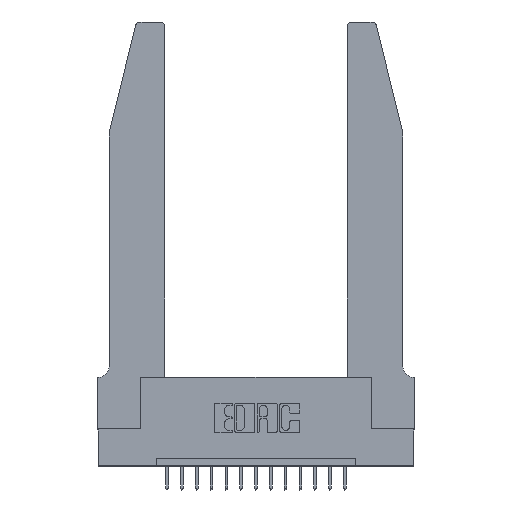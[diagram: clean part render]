
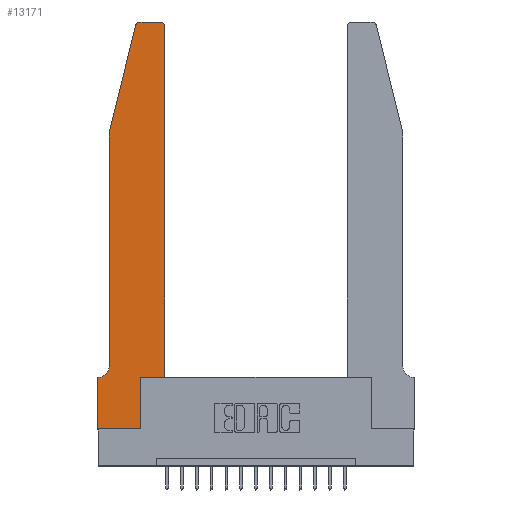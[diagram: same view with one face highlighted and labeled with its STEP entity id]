
A CAD part, top view. The second image highlights one B-rep face of the part: STEP entity #13171.
In plain terms, the highlighted planar face has unit normal (0, 0, 1).
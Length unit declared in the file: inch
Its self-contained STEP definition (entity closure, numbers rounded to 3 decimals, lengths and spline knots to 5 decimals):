
#63 = ORIENTED_EDGE ( 'NONE', *, *, #3996, .T. ) ;
#322 = FACE_OUTER_BOUND ( 'NONE', #7025, .T. ) ;
#660 = EDGE_CURVE ( 'NONE', #3453, #703, #4772, .T. ) ;
#703 = VERTEX_POINT ( 'NONE', #13868 ) ;
#1076 = VERTEX_POINT ( 'NONE', #10094 ) ;
#1338 = CARTESIAN_POINT ( 'NONE',  ( 0.0755, 2., 0.37 ) ) ;
#1634 = ORIENTED_EDGE ( 'NONE', *, *, #14730, .T. ) ;
#1838 = DIRECTION ( 'NONE',  ( 0., 1., 0. ) ) ;
#2089 = EDGE_CURVE ( 'NONE', #10853, #3168, #15451, .T. ) ;
#2152 = CARTESIAN_POINT ( 'NONE',  ( 0.4505, 0.35, 0.37 ) ) ;
#2156 = CARTESIAN_POINT ( 'NONE',  ( 0.4505, 0.35, 0.37 ) ) ;
#2313 = VECTOR ( 'NONE', #9971, 39.37008 ) ;
#2449 = DIRECTION ( 'NONE',  ( 0., 0., 1. ) ) ;
#2515 = LINE ( 'NONE', #1338, #14094 ) ;
#2856 = DIRECTION ( 'NONE',  ( 0., 0., 1. ) ) ;
#2957 = EDGE_CURVE ( 'NONE', #16217, #2970, #8934, .T. ) ;
#2970 = VERTEX_POINT ( 'NONE', #7116 ) ;
#3040 = PLANE ( 'NONE',  #16003 ) ;
#3168 = VERTEX_POINT ( 'NONE', #15044 ) ;
#3453 = VERTEX_POINT ( 'NONE', #18419 ) ;
#3845 = ORIENTED_EDGE ( 'NONE', *, *, #8795, .T. ) ;
#3909 = DIRECTION ( 'NONE',  ( 0., 0., 1. ) ) ;
#3985 = CARTESIAN_POINT ( 'NONE',  ( 0.0755, 0.35, 0.37 ) ) ;
#3996 = EDGE_CURVE ( 'NONE', #17017, #3453, #8462, .T. ) ;
#4078 = VECTOR ( 'NONE', #12708, 39.37008 ) ;
#4136 = DIRECTION ( 'NONE',  ( 0., -1., 0. ) ) ;
#4140 = LINE ( 'NONE', #13103, #18165 ) ;
#4772 = CIRCLE ( 'NONE', #15801, 0.03 ) ;
#5341 = EDGE_CURVE ( 'NONE', #1076, #16217, #13774, .T. ) ;
#5380 = CARTESIAN_POINT ( 'NONE',  ( 0.284, 2.72, 0.37 ) ) ;
#5930 = VECTOR ( 'NONE', #4136, 39.37008 ) ;
#5933 = DIRECTION ( 'NONE',  ( 1., 0., 0. ) ) ;
#6638 = DIRECTION ( 'NONE',  ( -1., 0., 0. ) ) ;
#6712 = CIRCLE ( 'NONE', #10894, 0.03 ) ;
#7025 = EDGE_LOOP ( 'NONE', ( #63, #17646, #1634, #7705, #10100, #3845, #17306, #12698, #14136, #13927, #10715, #9337 ) ) ;
#7116 = CARTESIAN_POINT ( 'NONE',  ( 0.4505, 2.72, 0.37 ) ) ;
#7169 = EDGE_CURVE ( 'NONE', #14162, #17605, #16854, .T. ) ;
#7196 = EDGE_CURVE ( 'NONE', #9338, #14162, #16417, .T. ) ;
#7284 = CARTESIAN_POINT ( 'NONE',  ( 0., 0.35, 0.37 ) ) ;
#7455 = CARTESIAN_POINT ( 'NONE',  ( 0.0755, 2., 0.37 ) ) ;
#7551 = CARTESIAN_POINT ( 'NONE',  ( 0.2605, 2.75, 0.37 ) ) ;
#7705 = ORIENTED_EDGE ( 'NONE', *, *, #7196, .T. ) ;
#8172 = DIRECTION ( 'NONE',  ( 1., 0., 0. ) ) ;
#8305 = DIRECTION ( 'NONE',  ( 1., 0., 0. ) ) ;
#8462 = LINE ( 'NONE', #7551, #4078 ) ;
#8795 = EDGE_CURVE ( 'NONE', #17605, #13874, #14074, .T. ) ;
#8934 = LINE ( 'NONE', #17096, #2313 ) ;
#9181 = VECTOR ( 'NONE', #8172, 39.37008 ) ;
#9291 = CARTESIAN_POINT ( 'NONE',  ( 0.0755, 2., 0.37 ) ) ;
#9337 = ORIENTED_EDGE ( 'NONE', *, *, #15269, .T. ) ;
#9338 = VERTEX_POINT ( 'NONE', #7455 ) ;
#9533 = CARTESIAN_POINT ( 'NONE',  ( 0.0055, 0.35, 0.37 ) ) ;
#9971 = DIRECTION ( 'NONE',  ( 0., 1., 0. ) ) ;
#10094 = CARTESIAN_POINT ( 'NONE',  ( 0.2865, 0.35, 0.37 ) ) ;
#10100 = ORIENTED_EDGE ( 'NONE', *, *, #7169, .T. ) ;
#10242 = CARTESIAN_POINT ( 'NONE',  ( 0., 0., 0.37 ) ) ;
#10715 = ORIENTED_EDGE ( 'NONE', *, *, #2957, .T. ) ;
#10853 = VERTEX_POINT ( 'NONE', #10242 ) ;
#10894 = AXIS2_PLACEMENT_3D ( 'NONE', #11143, #3909, #13817 ) ;
#11143 = CARTESIAN_POINT ( 'NONE',  ( 0.4205, 2.72, 0.37 ) ) ;
#11272 = CARTESIAN_POINT ( 'NONE',  ( 0.4205, 2.75, 0.37 ) ) ;
#11294 = DIRECTION ( 'NONE',  ( -0.239, -0.971, 0. ) ) ;
#11436 = CARTESIAN_POINT ( 'NONE',  ( 0., 0.35, 0.37 ) ) ;
#11869 = VECTOR ( 'NONE', #1838, 39.37008 ) ;
#11951 = AXIS2_PLACEMENT_3D ( 'NONE', #15025, #15149, #6638 ) ;
#12335 = LINE ( 'NONE', #14653, #11869 ) ;
#12698 = ORIENTED_EDGE ( 'NONE', *, *, #2089, .T. ) ;
#12708 = DIRECTION ( 'NONE',  ( -1., 0., 0. ) ) ;
#12768 = CARTESIAN_POINT ( 'NONE',  ( 0.0755, 0.42, 0.37 ) ) ;
#13103 = CARTESIAN_POINT ( 'NONE',  ( 0., 0., 0.37 ) ) ;
#13171 = ADVANCED_FACE ( 'NONE', ( #322 ), #3040, .T. ) ;
#13179 = VECTOR ( 'NONE', #18378, 39.37008 ) ;
#13774 = LINE ( 'NONE', #2152, #15765 ) ;
#13817 = DIRECTION ( 'NONE',  ( 1., 0., 0. ) ) ;
#13868 = CARTESIAN_POINT ( 'NONE',  ( 0.25487, 2.72718, 0.37 ) ) ;
#13874 = VERTEX_POINT ( 'NONE', #11436 ) ;
#13927 = ORIENTED_EDGE ( 'NONE', *, *, #5341, .T. ) ;
#14074 = LINE ( 'NONE', #3985, #13179 ) ;
#14094 = VECTOR ( 'NONE', #11294, 39.37008 ) ;
#14108 = CARTESIAN_POINT ( 'NONE',  ( 0., 0., 0.37 ) ) ;
#14136 = ORIENTED_EDGE ( 'NONE', *, *, #14348, .T. ) ;
#14162 = VERTEX_POINT ( 'NONE', #12768 ) ;
#14325 = EDGE_CURVE ( 'NONE', #13874, #10853, #4140, .T. ) ;
#14348 = EDGE_CURVE ( 'NONE', #3168, #1076, #12335, .T. ) ;
#14653 = CARTESIAN_POINT ( 'NONE',  ( 0.2865, 0.35, 0.37 ) ) ;
#14730 = EDGE_CURVE ( 'NONE', #703, #9338, #2515, .T. ) ;
#15025 = CARTESIAN_POINT ( 'NONE',  ( 0.0055, 0.42, 0.37 ) ) ;
#15044 = CARTESIAN_POINT ( 'NONE',  ( 0.2865, 0., 0.37 ) ) ;
#15149 = DIRECTION ( 'NONE',  ( 0., 0., -1. ) ) ;
#15269 = EDGE_CURVE ( 'NONE', #2970, #17017, #6712, .T. ) ;
#15451 = LINE ( 'NONE', #14108, #9181 ) ;
#15716 = DIRECTION ( 'NONE',  ( 0., -1., 0. ) ) ;
#15765 = VECTOR ( 'NONE', #18171, 39.37008 ) ;
#15801 = AXIS2_PLACEMENT_3D ( 'NONE', #5380, #2449, #8305 ) ;
#16003 = AXIS2_PLACEMENT_3D ( 'NONE', #7284, #2856, #5933 ) ;
#16217 = VERTEX_POINT ( 'NONE', #2156 ) ;
#16417 = LINE ( 'NONE', #9291, #5930 ) ;
#16854 = CIRCLE ( 'NONE', #11951, 0.07 ) ;
#17017 = VERTEX_POINT ( 'NONE', #11272 ) ;
#17096 = CARTESIAN_POINT ( 'NONE',  ( 0.4505, 0.35, 0.37 ) ) ;
#17306 = ORIENTED_EDGE ( 'NONE', *, *, #14325, .T. ) ;
#17605 = VERTEX_POINT ( 'NONE', #9533 ) ;
#17646 = ORIENTED_EDGE ( 'NONE', *, *, #660, .T. ) ;
#18165 = VECTOR ( 'NONE', #15716, 39.37008 ) ;
#18171 = DIRECTION ( 'NONE',  ( 1., 0., 0. ) ) ;
#18378 = DIRECTION ( 'NONE',  ( -1., 0., 0. ) ) ;
#18419 = CARTESIAN_POINT ( 'NONE',  ( 0.284, 2.75, 0.37 ) ) ;
